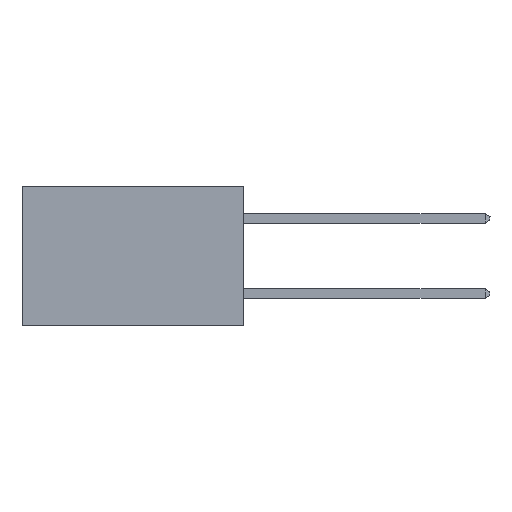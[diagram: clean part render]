
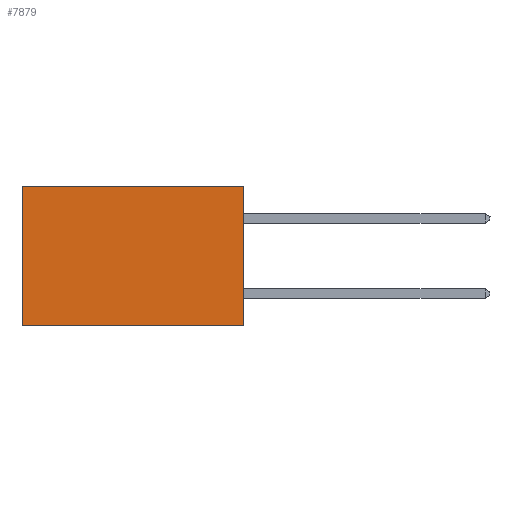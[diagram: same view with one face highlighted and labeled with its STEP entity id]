
A CAD part, left-side view. The second image highlights one B-rep face of the part: STEP entity #7879.
In plain terms, the highlighted planar face has unit normal (-1, 0, 0).
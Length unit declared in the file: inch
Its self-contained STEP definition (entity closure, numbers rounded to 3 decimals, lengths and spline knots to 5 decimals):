
#50 = LINE ( 'NONE', #15980, #9034 ) ;
#225 = FACE_OUTER_BOUND ( 'NONE', #18833, .T. ) ;
#303 = ORIENTED_EDGE ( 'NONE', *, *, #11004, .T. ) ;
#2246 = LINE ( 'NONE', #20210, #21888 ) ;
#2330 = ORIENTED_EDGE ( 'NONE', *, *, #20089, .F. ) ;
#2353 = CARTESIAN_POINT ( 'NONE',  ( 0.277, 0.59, -0.37 ) ) ;
#3292 = CARTESIAN_POINT ( 'NONE',  ( 0.277, 0., 0. ) ) ;
#4251 = ORIENTED_EDGE ( 'NONE', *, *, #14762, .F. ) ;
#4941 = CARTESIAN_POINT ( 'NONE',  ( 0.277, 0.59, 0. ) ) ;
#5880 = VECTOR ( 'NONE', #22726, 39.37008 ) ;
#5941 = AXIS2_PLACEMENT_3D ( 'NONE', #6527, #6505, #6475 ) ;
#6202 = CARTESIAN_POINT ( 'NONE',  ( 0.277, 0., -0.37 ) ) ;
#6475 = DIRECTION ( 'NONE',  ( 0., 0., -1. ) ) ;
#6505 = DIRECTION ( 'NONE',  ( 1., 0., 0. ) ) ;
#6527 = CARTESIAN_POINT ( 'NONE',  ( 0.277, 0., -0.37 ) ) ;
#6771 = PLANE ( 'NONE',  #5941 ) ;
#7879 = ADVANCED_FACE ( 'NONE', ( #225 ), #6771, .F. ) ;
#9034 = VECTOR ( 'NONE', #16069, 39.37008 ) ;
#9507 = CARTESIAN_POINT ( 'NONE',  ( 0.277, 0., -0.37 ) ) ;
#10944 = VECTOR ( 'NONE', #13613, 39.37008 ) ;
#11004 = EDGE_CURVE ( 'NONE', #13751, #20281, #50, .T. ) ;
#11250 = VERTEX_POINT ( 'NONE', #3292 ) ;
#11536 = LINE ( 'NONE', #22975, #10944 ) ;
#13613 = DIRECTION ( 'NONE',  ( 0., 0., -1. ) ) ;
#13751 = VERTEX_POINT ( 'NONE', #4941 ) ;
#13852 = ORIENTED_EDGE ( 'NONE', *, *, #14459, .T. ) ;
#14459 = EDGE_CURVE ( 'NONE', #11250, #13751, #2246, .T. ) ;
#14762 = EDGE_CURVE ( 'NONE', #11250, #19058, #11536, .T. ) ;
#15432 = LINE ( 'NONE', #9507, #5880 ) ;
#15980 = CARTESIAN_POINT ( 'NONE',  ( 0.277, 0.59, -0.37 ) ) ;
#16069 = DIRECTION ( 'NONE',  ( 0., 0., -1. ) ) ;
#18833 = EDGE_LOOP ( 'NONE', ( #303, #2330, #4251, #13852 ) ) ;
#19058 = VERTEX_POINT ( 'NONE', #6202 ) ;
#20089 = EDGE_CURVE ( 'NONE', #19058, #20281, #15432, .T. ) ;
#20210 = CARTESIAN_POINT ( 'NONE',  ( 0.277, 0., 0. ) ) ;
#20281 = VERTEX_POINT ( 'NONE', #2353 ) ;
#20285 = DIRECTION ( 'NONE',  ( 0., 1., 0. ) ) ;
#21888 = VECTOR ( 'NONE', #20285, 39.37008 ) ;
#22726 = DIRECTION ( 'NONE',  ( 0., 1., 0. ) ) ;
#22975 = CARTESIAN_POINT ( 'NONE',  ( 0.277, 0., -0.37 ) ) ;
